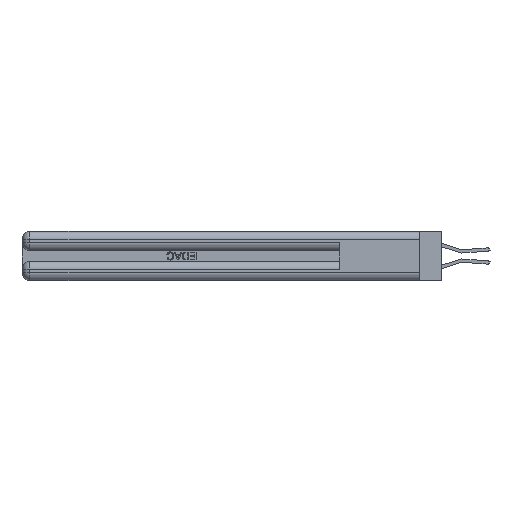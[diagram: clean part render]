
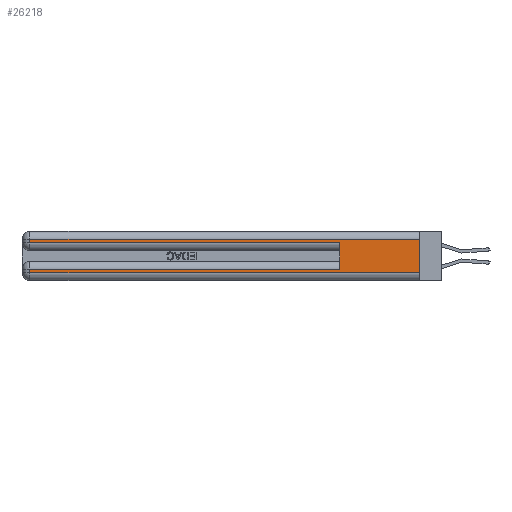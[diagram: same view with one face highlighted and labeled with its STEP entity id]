
A CAD part, left-side view. The second image highlights one B-rep face of the part: STEP entity #26218.
In plain terms, the highlighted planar face has unit normal (-1, 0, 0).
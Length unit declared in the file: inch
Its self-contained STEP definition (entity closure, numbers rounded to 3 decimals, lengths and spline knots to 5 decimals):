
#2421 = EDGE_CURVE ( 'NONE', #16127, #21721, #5062, .T. ) ;
#2884 = VECTOR ( 'NONE', #26770, 39.37008 ) ;
#3747 = LINE ( 'NONE', #30937, #23238 ) ;
#4500 = CARTESIAN_POINT ( 'NONE',  ( 0., 0.6, 0.145 ) ) ;
#5062 = LINE ( 'NONE', #42487, #15651 ) ;
#5928 = LINE ( 'NONE', #4500, #27469 ) ;
#6164 = DIRECTION ( 'NONE',  ( 0., 0., -1. ) ) ;
#6820 = CARTESIAN_POINT ( 'NONE',  ( 0., 0.6, 0.085 ) ) ;
#6866 = EDGE_CURVE ( 'NONE', #13438, #46658, #37050, .T. ) ;
#7565 = LINE ( 'NONE', #16822, #26425 ) ;
#7663 = CARTESIAN_POINT ( 'NONE',  ( 0., 0., 0.31 ) ) ;
#8491 = CARTESIAN_POINT ( 'NONE',  ( 0., 0., 0.06 ) ) ;
#8514 = DIRECTION ( 'NONE',  ( 0., 0., -1. ) ) ;
#8741 = ORIENTED_EDGE ( 'NONE', *, *, #30631, .T. ) ;
#9402 = PLANE ( 'NONE',  #37593 ) ;
#9804 = ORIENTED_EDGE ( 'NONE', *, *, #26233, .T. ) ;
#10275 = ORIENTED_EDGE ( 'NONE', *, *, #6866, .T. ) ;
#10527 = LINE ( 'NONE', #7663, #2884 ) ;
#13438 = VERTEX_POINT ( 'NONE', #44322 ) ;
#13918 = CARTESIAN_POINT ( 'NONE',  ( 0., 2.94, 0.285 ) ) ;
#14482 = EDGE_CURVE ( 'NONE', #34977, #38736, #17293, .T. ) ;
#14677 = CARTESIAN_POINT ( 'NONE',  ( 0., 0., 0.31 ) ) ;
#15651 = VECTOR ( 'NONE', #24828, 39.37008 ) ;
#16127 = VERTEX_POINT ( 'NONE', #13918 ) ;
#16822 = CARTESIAN_POINT ( 'NONE',  ( 0., 2.94, 0.37 ) ) ;
#17293 = LINE ( 'NONE', #39396, #18472 ) ;
#17942 = ORIENTED_EDGE ( 'NONE', *, *, #27484, .F. ) ;
#18472 = VECTOR ( 'NONE', #20736, 39.37008 ) ;
#19904 = CARTESIAN_POINT ( 'NONE',  ( 0., 0.6, 0.285 ) ) ;
#20367 = VERTEX_POINT ( 'NONE', #37714 ) ;
#20431 = DIRECTION ( 'NONE',  ( 0., 0., -1. ) ) ;
#20736 = DIRECTION ( 'NONE',  ( 0., 1., 0. ) ) ;
#21721 = VERTEX_POINT ( 'NONE', #19904 ) ;
#22179 = ORIENTED_EDGE ( 'NONE', *, *, #39304, .T. ) ;
#22938 = VECTOR ( 'NONE', #6164, 39.37008 ) ;
#23238 = VECTOR ( 'NONE', #8514, 39.37008 ) ;
#23363 = CARTESIAN_POINT ( 'NONE',  ( 0., 2.94, 0.085 ) ) ;
#23834 = CARTESIAN_POINT ( 'NONE',  ( 0., 0., 0.37 ) ) ;
#24828 = DIRECTION ( 'NONE',  ( 0., -1., 0. ) ) ;
#26218 = ADVANCED_FACE ( 'NONE', ( #31741 ), #9402, .F. ) ;
#26233 = EDGE_CURVE ( 'NONE', #38736, #13438, #7565, .T. ) ;
#26408 = VECTOR ( 'NONE', #37505, 39.37008 ) ;
#26425 = VECTOR ( 'NONE', #28068, 39.37008 ) ;
#26770 = DIRECTION ( 'NONE',  ( 0., 1., 0. ) ) ;
#27469 = VECTOR ( 'NONE', #31264, 39.37008 ) ;
#27484 = EDGE_CURVE ( 'NONE', #48474, #46658, #46503, .T. ) ;
#28068 = DIRECTION ( 'NONE',  ( 0., 0., -1. ) ) ;
#30631 = EDGE_CURVE ( 'NONE', #20367, #16127, #3747, .T. ) ;
#30937 = CARTESIAN_POINT ( 'NONE',  ( 0., 2.94, 0.37 ) ) ;
#31264 = DIRECTION ( 'NONE',  ( 0., 0., 1. ) ) ;
#31339 = ORIENTED_EDGE ( 'NONE', *, *, #14482, .T. ) ;
#31741 = FACE_OUTER_BOUND ( 'NONE', #48535, .T. ) ;
#31833 = DIRECTION ( 'NONE',  ( 1., 0., 0. ) ) ;
#34977 = VERTEX_POINT ( 'NONE', #6820 ) ;
#37050 = LINE ( 'NONE', #48634, #26408 ) ;
#37505 = DIRECTION ( 'NONE',  ( 0., -1., 0. ) ) ;
#37583 = ORIENTED_EDGE ( 'NONE', *, *, #46752, .F. ) ;
#37593 = AXIS2_PLACEMENT_3D ( 'NONE', #46930, #31833, #20431 ) ;
#37714 = CARTESIAN_POINT ( 'NONE',  ( 0., 2.94, 0.31 ) ) ;
#38736 = VERTEX_POINT ( 'NONE', #23363 ) ;
#39304 = EDGE_CURVE ( 'NONE', #48474, #20367, #10527, .T. ) ;
#39396 = CARTESIAN_POINT ( 'NONE',  ( 0., 0., 0.085 ) ) ;
#42487 = CARTESIAN_POINT ( 'NONE',  ( 0., 0., 0.285 ) ) ;
#44237 = ORIENTED_EDGE ( 'NONE', *, *, #2421, .T. ) ;
#44322 = CARTESIAN_POINT ( 'NONE',  ( 0., 2.94, 0.06 ) ) ;
#46503 = LINE ( 'NONE', #23834, #22938 ) ;
#46658 = VERTEX_POINT ( 'NONE', #8491 ) ;
#46752 = EDGE_CURVE ( 'NONE', #34977, #21721, #5928, .T. ) ;
#46930 = CARTESIAN_POINT ( 'NONE',  ( 0., 0., 0.37 ) ) ;
#48474 = VERTEX_POINT ( 'NONE', #14677 ) ;
#48535 = EDGE_LOOP ( 'NONE', ( #17942, #22179, #8741, #44237, #37583, #31339, #9804, #10275 ) ) ;
#48634 = CARTESIAN_POINT ( 'NONE',  ( 0., 0., 0.06 ) ) ;
